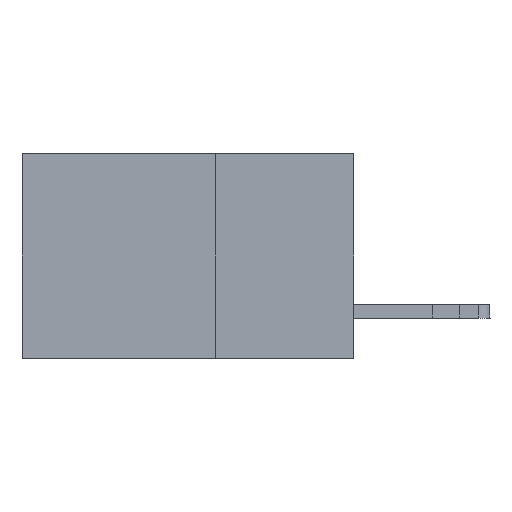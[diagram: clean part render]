
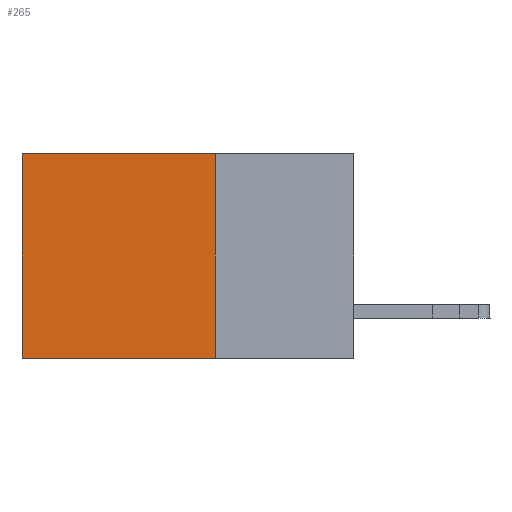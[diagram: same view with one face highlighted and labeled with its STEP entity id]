
A CAD part, left-side view. The second image highlights one B-rep face of the part: STEP entity #265.
In plain terms, the highlighted planar face has unit normal (-1, 0, 0).
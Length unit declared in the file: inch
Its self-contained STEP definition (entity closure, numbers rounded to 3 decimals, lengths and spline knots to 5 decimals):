
#26 = VECTOR ( 'NONE', #25681, 39.37008 ) ;
#265 = ADVANCED_FACE ( 'NONE', ( #15633 ), #1413, .F. ) ;
#334 = VERTEX_POINT ( 'NONE', #29114 ) ;
#758 = CARTESIAN_POINT ( 'NONE',  ( 0.2875, 0.25, 0. ) ) ;
#790 = DIRECTION ( 'NONE',  ( 0., 1., 0. ) ) ;
#1413 = PLANE ( 'NONE',  #21356 ) ;
#4462 = DIRECTION ( 'NONE',  ( 0., 0., -1. ) ) ;
#7049 = EDGE_CURVE ( 'NONE', #25692, #334, #11509, .T. ) ;
#7842 = CARTESIAN_POINT ( 'NONE',  ( 0.2875, 0.6, 0. ) ) ;
#9425 = EDGE_CURVE ( 'NONE', #25282, #19245, #28557, .T. ) ;
#11454 = ORIENTED_EDGE ( 'NONE', *, *, #15932, .F. ) ;
#11470 = ORIENTED_EDGE ( 'NONE', *, *, #7049, .T. ) ;
#11509 = LINE ( 'NONE', #24901, #23994 ) ;
#12626 = DIRECTION ( 'NONE',  ( 0., 0., -1. ) ) ;
#14474 = CARTESIAN_POINT ( 'NONE',  ( 0.2875, 0.25, -0.37 ) ) ;
#14979 = CARTESIAN_POINT ( 'NONE',  ( 0.2875, 0.25, 0. ) ) ;
#15633 = FACE_OUTER_BOUND ( 'NONE', #27874, .T. ) ;
#15932 = EDGE_CURVE ( 'NONE', #19245, #334, #22579, .T. ) ;
#16070 = ORIENTED_EDGE ( 'NONE', *, *, #20657, .T. ) ;
#17735 = CARTESIAN_POINT ( 'NONE',  ( 0.2875, 0.25, -0.37 ) ) ;
#19245 = VERTEX_POINT ( 'NONE', #17735 ) ;
#19571 = DIRECTION ( 'NONE',  ( 1., 0., 0. ) ) ;
#20657 = EDGE_CURVE ( 'NONE', #25282, #25692, #23984, .T. ) ;
#21356 = AXIS2_PLACEMENT_3D ( 'NONE', #14979, #19571, #24270 ) ;
#22579 = LINE ( 'NONE', #14474, #29439 ) ;
#23984 = LINE ( 'NONE', #28352, #26 ) ;
#23994 = VECTOR ( 'NONE', #4462, 39.37008 ) ;
#24270 = DIRECTION ( 'NONE',  ( 0., 0., -1. ) ) ;
#24901 = CARTESIAN_POINT ( 'NONE',  ( 0.2875, 0.6, 0. ) ) ;
#25258 = VECTOR ( 'NONE', #12626, 39.37008 ) ;
#25282 = VERTEX_POINT ( 'NONE', #758 ) ;
#25681 = DIRECTION ( 'NONE',  ( 0., 1., 0. ) ) ;
#25692 = VERTEX_POINT ( 'NONE', #7842 ) ;
#26032 = CARTESIAN_POINT ( 'NONE',  ( 0.2875, 0.25, 0. ) ) ;
#27874 = EDGE_LOOP ( 'NONE', ( #11470, #11454, #28753, #16070 ) ) ;
#28352 = CARTESIAN_POINT ( 'NONE',  ( 0.2875, 0.25, 0. ) ) ;
#28557 = LINE ( 'NONE', #26032, #25258 ) ;
#28753 = ORIENTED_EDGE ( 'NONE', *, *, #9425, .F. ) ;
#29114 = CARTESIAN_POINT ( 'NONE',  ( 0.2875, 0.6, -0.37 ) ) ;
#29439 = VECTOR ( 'NONE', #790, 39.37008 ) ;
